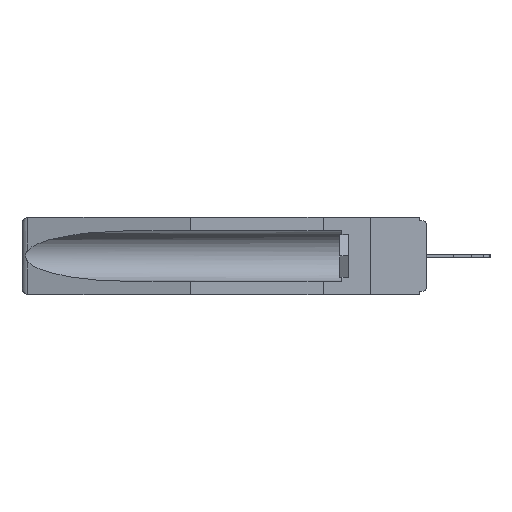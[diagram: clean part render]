
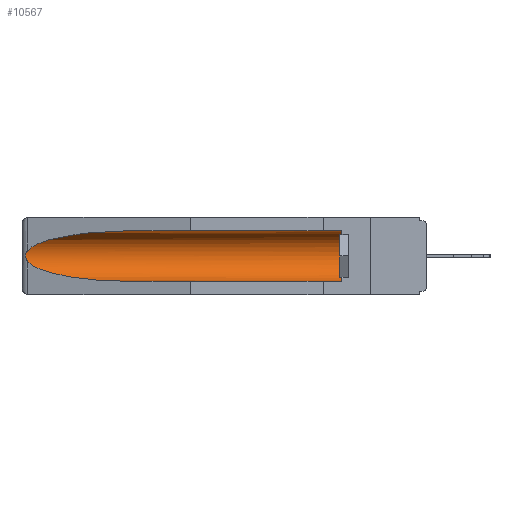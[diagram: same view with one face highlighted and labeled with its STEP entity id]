
A CAD part, left-side view. The second image highlights one B-rep face of the part: STEP entity #10567.
In plain terms, the highlighted cylindrical face has radius 2.857 mm (diameter 5.715 mm), a partial arc.
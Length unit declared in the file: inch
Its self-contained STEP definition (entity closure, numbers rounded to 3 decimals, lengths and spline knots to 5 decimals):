
#32 = CARTESIAN_POINT ( 'NONE',  ( 0.155, 0.126, -0.1715 ) ) ;
#211 = CYLINDRICAL_SURFACE ( 'NONE', #3379, 0.1125 ) ;
#2368 = DIRECTION ( 'NONE',  ( 0., 0., 1. ) ) ;
#2980 = EDGE_CURVE ( 'NONE', #7400, #28115, #21074, .T. ) ;
#3119 = CARTESIAN_POINT ( 'NONE',  ( 0.25451, 1.48313, -0.09465 ) ) ;
#3379 = AXIS2_PLACEMENT_3D ( 'NONE', #5758, #21827, #24138 ) ;
#3959 = DIRECTION ( 'NONE',  ( 0., 1., 0. ) ) ;
#4712 = EDGE_CURVE ( 'NONE', #28986, #21143, #18159, .T. ) ;
#4989 = EDGE_CURVE ( 'NONE', #28115, #6784, #27330, .T. ) ;
#5758 = CARTESIAN_POINT ( 'NONE',  ( 0.155, -0.30754, -0.1715 ) ) ;
#6275 = CARTESIAN_POINT ( 'NONE',  ( 0.155, -0.30754, -0.284 ) ) ;
#6331 = FACE_OUTER_BOUND ( 'NONE', #10136, .T. ) ;
#6784 = VERTEX_POINT ( 'NONE', #22715 ) ;
#7287 = CARTESIAN_POINT ( 'NONE',  ( 0.26537, 1.52718, -0.19328 ) ) ;
#7372 = CARTESIAN_POINT ( 'NONE',  ( 0.26597, 1.52961, -0.15275 ) ) ;
#7400 = VERTEX_POINT ( 'NONE', #14006 ) ;
#8323 = CARTESIAN_POINT ( 'NONE',  ( 0.2673, 1.53269, -0.17917 ) ) ;
#9690 = CARTESIAN_POINT ( 'NONE',  ( 0.26654, 1.53092, -0.15636 ) ) ;
#10136 = EDGE_LOOP ( 'NONE', ( #25186, #10769, #23780, #22321, #20957, #17450 ) ) ;
#10365 = CARTESIAN_POINT ( 'NONE',  ( 0.2675, 1.53308, -0.17534 ) ) ;
#10567 = ADVANCED_FACE ( 'NONE', ( #6331 ), #211, .F. ) ;
#10769 = ORIENTED_EDGE ( 'NONE', *, *, #2980, .T. ) ;
#11375 =( BOUNDED_CURVE ( )  B_SPLINE_CURVE ( 3, ( #21011, #23333, #3119, #19214 ),
 .UNSPECIFIED., .F., .F. ) 
 B_SPLINE_CURVE_WITH_KNOTS ( ( 4, 4 ),
 ( 4.71239, 6.08839 ),
 .UNSPECIFIED. ) 
 CURVE ( )  GEOMETRIC_REPRESENTATION_ITEM ( )  RATIONAL_B_SPLINE_CURVE ( ( 1., 0.848, 0.848, 1. ) ) 
 REPRESENTATION_ITEM ( '' )  );
#11466 = CARTESIAN_POINT ( 'NONE',  ( 0.2673, 1.5327, -0.16383 ) ) ;
#11817 = CARTESIAN_POINT ( 'NONE',  ( 0.2675, 1.53308, -0.16763 ) ) ;
#12746 = CARTESIAN_POINT ( 'NONE',  ( 0.25451, 1.48313, -0.24835 ) ) ;
#14006 = CARTESIAN_POINT ( 'NONE',  ( 0.26537, 1.52718, -0.14972 ) ) ;
#15262 = EDGE_CURVE ( 'NONE', #20973, #28986, #17389, .T. ) ;
#16051 = EDGE_CURVE ( 'NONE', #21143, #7400, #11375, .T. ) ;
#16099 = DIRECTION ( 'NONE',  ( 0., -1., 0. ) ) ;
#17016 = CARTESIAN_POINT ( 'NONE',  ( 0.155, -0.30754, -0.059 ) ) ;
#17047 = DIRECTION ( 'NONE',  ( 0., 1., 0. ) ) ;
#17389 = CIRCLE ( 'NONE', #18871, 0.1125 ) ;
#17450 = ORIENTED_EDGE ( 'NONE', *, *, #4712, .T. ) ;
#18159 = LINE ( 'NONE', #17016, #18882 ) ;
#18610 = CARTESIAN_POINT ( 'NONE',  ( 0.155, 0.126, -0.284 ) ) ;
#18871 = AXIS2_PLACEMENT_3D ( 'NONE', #32, #16099, #2368 ) ;
#18882 = VECTOR ( 'NONE', #17047, 39.37008 ) ;
#19214 = CARTESIAN_POINT ( 'NONE',  ( 0.26537, 1.52718, -0.14972 ) ) ;
#20447 = CARTESIAN_POINT ( 'NONE',  ( 0.26537, 1.52718, -0.19328 ) ) ;
#20957 = ORIENTED_EDGE ( 'NONE', *, *, #15262, .T. ) ;
#20973 = VERTEX_POINT ( 'NONE', #18610 ) ;
#21011 = CARTESIAN_POINT ( 'NONE',  ( 0.155, 1.07973, -0.059 ) ) ;
#21064 = CARTESIAN_POINT ( 'NONE',  ( 0.155, 0.126, -0.059 ) ) ;
#21074 = B_SPLINE_CURVE_WITH_KNOTS ( 'NONE', 3,
 ( #24968, #7372, #9690, #11466, #11817, #10365, #8323, #24183, #27943, #27601 ),
 .UNSPECIFIED., .F., .F.,
 ( 4, 2, 2, 2, 4 ),
 ( 0., 0.00029, 0.00058, 0.00087, 0.00117 ),
 .UNSPECIFIED. ) ;
#21143 = VERTEX_POINT ( 'NONE', #24341 ) ;
#21606 = LINE ( 'NONE', #6275, #25547 ) ;
#21827 = DIRECTION ( 'NONE',  ( 0., 1., 0. ) ) ;
#22321 = ORIENTED_EDGE ( 'NONE', *, *, #26679, .F. ) ;
#22715 = CARTESIAN_POINT ( 'NONE',  ( 0.155, 1.07973, -0.284 ) ) ;
#23333 = CARTESIAN_POINT ( 'NONE',  ( 0.21114, 1.30732, -0.059 ) ) ;
#23780 = ORIENTED_EDGE ( 'NONE', *, *, #4989, .T. ) ;
#24098 = CARTESIAN_POINT ( 'NONE',  ( 0.155, 1.07973, -0.284 ) ) ;
#24138 = DIRECTION ( 'NONE',  ( 0., 0., 1. ) ) ;
#24183 = CARTESIAN_POINT ( 'NONE',  ( 0.26655, 1.53094, -0.18657 ) ) ;
#24341 = CARTESIAN_POINT ( 'NONE',  ( 0.155, 1.07973, -0.059 ) ) ;
#24968 = CARTESIAN_POINT ( 'NONE',  ( 0.26537, 1.52718, -0.14972 ) ) ;
#25186 = ORIENTED_EDGE ( 'NONE', *, *, #16051, .T. ) ;
#25547 = VECTOR ( 'NONE', #3959, 39.37008 ) ;
#25941 = CARTESIAN_POINT ( 'NONE',  ( 0.21114, 1.30732, -0.284 ) ) ;
#26679 = EDGE_CURVE ( 'NONE', #20973, #6784, #21606, .T. ) ;
#27330 =( BOUNDED_CURVE ( )  B_SPLINE_CURVE ( 3, ( #20447, #12746, #25941, #24098 ),
 .UNSPECIFIED., .F., .F. ) 
 B_SPLINE_CURVE_WITH_KNOTS ( ( 4, 4 ),
 ( 0.1948, 1.5708 ),
 .UNSPECIFIED. ) 
 CURVE ( )  GEOMETRIC_REPRESENTATION_ITEM ( )  RATIONAL_B_SPLINE_CURVE ( ( 1., 0.848, 0.848, 1. ) ) 
 REPRESENTATION_ITEM ( '' )  );
#27601 = CARTESIAN_POINT ( 'NONE',  ( 0.26537, 1.52718, -0.19328 ) ) ;
#27943 = CARTESIAN_POINT ( 'NONE',  ( 0.26597, 1.5296, -0.19026 ) ) ;
#28115 = VERTEX_POINT ( 'NONE', #7287 ) ;
#28986 = VERTEX_POINT ( 'NONE', #21064 ) ;
